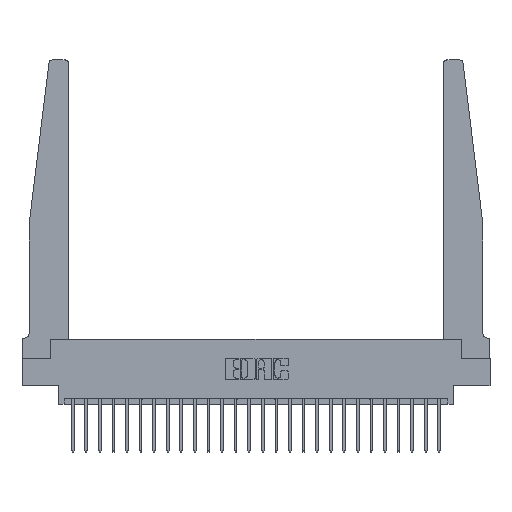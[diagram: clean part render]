
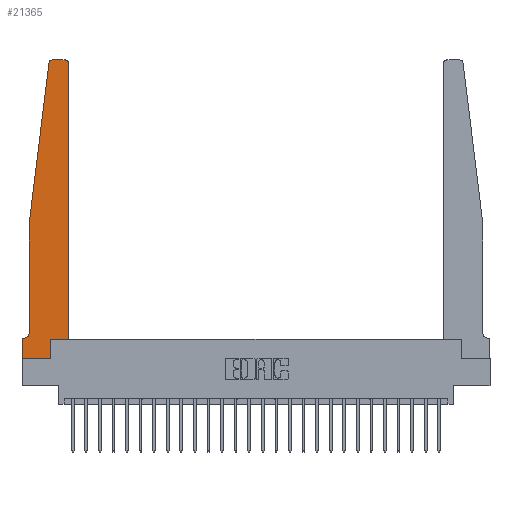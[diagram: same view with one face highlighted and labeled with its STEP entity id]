
A CAD part, top view. The second image highlights one B-rep face of the part: STEP entity #21365.
In plain terms, the highlighted planar face has unit normal (0, 0, 1).
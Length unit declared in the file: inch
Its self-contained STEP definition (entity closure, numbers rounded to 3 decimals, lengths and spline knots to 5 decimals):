
#193 = FACE_OUTER_BOUND ( 'NONE', #17409, .T. ) ;
#212 = ORIENTED_EDGE ( 'NONE', *, *, #19053, .T. ) ;
#500 = DIRECTION ( 'NONE',  ( 1., 0., 0. ) ) ;
#518 = DIRECTION ( 'NONE',  ( 0., 1., 0. ) ) ;
#773 = VERTEX_POINT ( 'NONE', #4415 ) ;
#908 = LINE ( 'NONE', #20270, #8499 ) ;
#1592 = LINE ( 'NONE', #5502, #15591 ) ;
#1881 = ORIENTED_EDGE ( 'NONE', *, *, #2191, .T. ) ;
#2191 = EDGE_CURVE ( 'NONE', #22583, #16235, #1592, .T. ) ;
#2205 = CARTESIAN_POINT ( 'NONE',  ( 0., 0., 0.37 ) ) ;
#2571 = VERTEX_POINT ( 'NONE', #14634 ) ;
#3139 = AXIS2_PLACEMENT_3D ( 'NONE', #25179, #17332, #22883 ) ;
#3301 = VERTEX_POINT ( 'NONE', #5584 ) ;
#3429 = ORIENTED_EDGE ( 'NONE', *, *, #5965, .T. ) ;
#3430 = LINE ( 'NONE', #13605, #21690 ) ;
#3838 = LINE ( 'NONE', #4083, #17380 ) ;
#3957 = DIRECTION ( 'NONE',  ( 1., 0., 0. ) ) ;
#4002 = LINE ( 'NONE', #2205, #6392 ) ;
#4083 = CARTESIAN_POINT ( 'NONE',  ( 0.25, 2.75, 0.37 ) ) ;
#4346 = CIRCLE ( 'NONE', #3139, 0.05 ) ;
#4415 = CARTESIAN_POINT ( 'NONE',  ( 0.065, 1.25, 0.37 ) ) ;
#4433 = ORIENTED_EDGE ( 'NONE', *, *, #8850, .T. ) ;
#4477 = CARTESIAN_POINT ( 'NONE',  ( 0.395, 2.72, 0.37 ) ) ;
#4877 = CARTESIAN_POINT ( 'NONE',  ( 0.27653, 2.72, 0.37 ) ) ;
#5073 = VERTEX_POINT ( 'NONE', #10333 ) ;
#5211 = AXIS2_PLACEMENT_3D ( 'NONE', #4477, #12326, #16764 ) ;
#5246 = VERTEX_POINT ( 'NONE', #9634 ) ;
#5502 = CARTESIAN_POINT ( 'NONE',  ( 0., 0., 0.37 ) ) ;
#5576 = VECTOR ( 'NONE', #9816, 39.37008 ) ;
#5584 = CARTESIAN_POINT ( 'NONE',  ( 0.24675, 2.72367, 0.37 ) ) ;
#5797 = CIRCLE ( 'NONE', #7436, 0.03 ) ;
#5965 = EDGE_CURVE ( 'NONE', #16235, #5246, #4002, .T. ) ;
#6039 = DIRECTION ( 'NONE',  ( 0., 0., 1. ) ) ;
#6377 = VERTEX_POINT ( 'NONE', #21422 ) ;
#6392 = VECTOR ( 'NONE', #500, 39.37008 ) ;
#6706 = VECTOR ( 'NONE', #15638, 39.37008 ) ;
#6880 = VERTEX_POINT ( 'NONE', #15744 ) ;
#7062 = EDGE_CURVE ( 'NONE', #6880, #2571, #22087, .T. ) ;
#7146 = VERTEX_POINT ( 'NONE', #24999 ) ;
#7384 = ORIENTED_EDGE ( 'NONE', *, *, #13287, .T. ) ;
#7436 = AXIS2_PLACEMENT_3D ( 'NONE', #4877, #14700, #14978 ) ;
#7507 = EDGE_CURVE ( 'NONE', #7146, #6880, #908, .T. ) ;
#8087 = PLANE ( 'NONE',  #20679 ) ;
#8499 = VECTOR ( 'NONE', #518, 39.37008 ) ;
#8850 = EDGE_CURVE ( 'NONE', #24681, #6377, #4346, .T. ) ;
#9122 = CARTESIAN_POINT ( 'NONE',  ( 0.065, 0.1875, 0.37 ) ) ;
#9634 = CARTESIAN_POINT ( 'NONE',  ( 0.2605, 0., 0.37 ) ) ;
#9816 = DIRECTION ( 'NONE',  ( 0., -1., 0. ) ) ;
#9894 = ORIENTED_EDGE ( 'NONE', *, *, #22301, .T. ) ;
#9896 = ORIENTED_EDGE ( 'NONE', *, *, #11519, .T. ) ;
#9916 = LINE ( 'NONE', #23241, #6706 ) ;
#9974 = DIRECTION ( 'NONE',  ( 0., -1., 0. ) ) ;
#10333 = CARTESIAN_POINT ( 'NONE',  ( 0.2605, 0.18, 0.37 ) ) ;
#10362 = CARTESIAN_POINT ( 'NONE',  ( 0., 0.1875, 0.37 ) ) ;
#11485 = CARTESIAN_POINT ( 'NONE',  ( 0.27653, 2.75, 0.37 ) ) ;
#11519 = EDGE_CURVE ( 'NONE', #2571, #21876, #3838, .T. ) ;
#11950 = DIRECTION ( 'NONE',  ( -1., 0., 0. ) ) ;
#12326 = DIRECTION ( 'NONE',  ( 0., 0., 1. ) ) ;
#13246 = LINE ( 'NONE', #9122, #23001 ) ;
#13287 = EDGE_CURVE ( 'NONE', #3301, #773, #3430, .T. ) ;
#13605 = CARTESIAN_POINT ( 'NONE',  ( 0.065, 1.25, 0.37 ) ) ;
#13818 = CARTESIAN_POINT ( 'NONE',  ( 0., 0., 0.37 ) ) ;
#14634 = CARTESIAN_POINT ( 'NONE',  ( 0.395, 2.75, 0.37 ) ) ;
#14700 = DIRECTION ( 'NONE',  ( 0., 0., 1. ) ) ;
#14978 = DIRECTION ( 'NONE',  ( 1., 0., 0. ) ) ;
#15284 = LINE ( 'NONE', #23138, #5576 ) ;
#15591 = VECTOR ( 'NONE', #9974, 39.37008 ) ;
#15620 = ORIENTED_EDGE ( 'NONE', *, *, #7507, .T. ) ;
#15638 = DIRECTION ( 'NONE',  ( 0., 1., 0. ) ) ;
#15698 = DIRECTION ( 'NONE',  ( -0.122, -0.992, 0. ) ) ;
#15744 = CARTESIAN_POINT ( 'NONE',  ( 0.425, 2.72, 0.37 ) ) ;
#16235 = VERTEX_POINT ( 'NONE', #13818 ) ;
#16596 = ORIENTED_EDGE ( 'NONE', *, *, #18658, .T. ) ;
#16646 = DIRECTION ( 'NONE',  ( 1., 0., 0. ) ) ;
#16764 = DIRECTION ( 'NONE',  ( 1., 0., 0. ) ) ;
#16784 = LINE ( 'NONE', #18694, #18642 ) ;
#17025 = DIRECTION ( 'NONE',  ( -1., 0., 0. ) ) ;
#17332 = DIRECTION ( 'NONE',  ( 0., 0., -1. ) ) ;
#17380 = VECTOR ( 'NONE', #11950, 39.37008 ) ;
#17409 = EDGE_LOOP ( 'NONE', ( #9896, #17932, #7384, #212, #4433, #16596, #1881, #3429, #21337, #9894, #15620, #24378 ) ) ;
#17920 = CARTESIAN_POINT ( 'NONE',  ( 0., 0.1875, 0.37 ) ) ;
#17932 = ORIENTED_EDGE ( 'NONE', *, *, #19740, .T. ) ;
#18642 = VECTOR ( 'NONE', #16646, 39.37008 ) ;
#18658 = EDGE_CURVE ( 'NONE', #6377, #22583, #13246, .T. ) ;
#18694 = CARTESIAN_POINT ( 'NONE',  ( 0.425, 0.18, 0.37 ) ) ;
#19053 = EDGE_CURVE ( 'NONE', #773, #24681, #15284, .T. ) ;
#19740 = EDGE_CURVE ( 'NONE', #21876, #3301, #5797, .T. ) ;
#20270 = CARTESIAN_POINT ( 'NONE',  ( 0.425, 0.18, 0.37 ) ) ;
#20679 = AXIS2_PLACEMENT_3D ( 'NONE', #17920, #6039, #3957 ) ;
#21337 = ORIENTED_EDGE ( 'NONE', *, *, #22099, .T. ) ;
#21365 = ADVANCED_FACE ( 'NONE', ( #193 ), #8087, .T. ) ;
#21422 = CARTESIAN_POINT ( 'NONE',  ( 0.015, 0.1875, 0.37 ) ) ;
#21690 = VECTOR ( 'NONE', #15698, 39.37008 ) ;
#21876 = VERTEX_POINT ( 'NONE', #11485 ) ;
#22087 = CIRCLE ( 'NONE', #5211, 0.03 ) ;
#22099 = EDGE_CURVE ( 'NONE', #5246, #5073, #9916, .T. ) ;
#22301 = EDGE_CURVE ( 'NONE', #5073, #7146, #16784, .T. ) ;
#22583 = VERTEX_POINT ( 'NONE', #10362 ) ;
#22843 = CARTESIAN_POINT ( 'NONE',  ( 0.065, 0.2375, 0.37 ) ) ;
#22883 = DIRECTION ( 'NONE',  ( -1., 0., 0. ) ) ;
#23001 = VECTOR ( 'NONE', #17025, 39.37008 ) ;
#23138 = CARTESIAN_POINT ( 'NONE',  ( 0.065, 1.25, 0.37 ) ) ;
#23241 = CARTESIAN_POINT ( 'NONE',  ( 0.2605, 0.18, 0.37 ) ) ;
#24378 = ORIENTED_EDGE ( 'NONE', *, *, #7062, .T. ) ;
#24681 = VERTEX_POINT ( 'NONE', #22843 ) ;
#24999 = CARTESIAN_POINT ( 'NONE',  ( 0.425, 0.18, 0.37 ) ) ;
#25179 = CARTESIAN_POINT ( 'NONE',  ( 0.015, 0.2375, 0.37 ) ) ;
